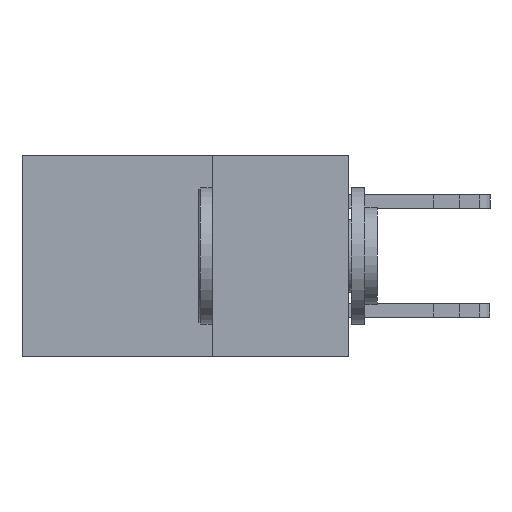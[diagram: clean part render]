
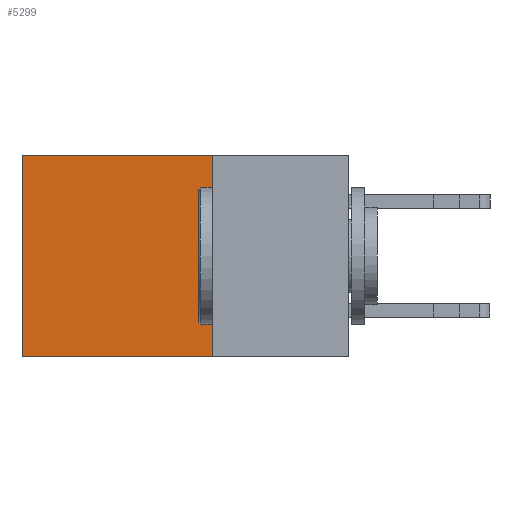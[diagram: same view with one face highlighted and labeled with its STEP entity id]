
A CAD part, left-side view. The second image highlights one B-rep face of the part: STEP entity #5299.
In plain terms, the highlighted planar face has unit normal (-1, 0, 0).
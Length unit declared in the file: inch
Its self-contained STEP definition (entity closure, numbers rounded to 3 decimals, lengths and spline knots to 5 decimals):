
#63 = CARTESIAN_POINT ( 'NONE',  ( 0.298, 0.6, -0.37 ) ) ;
#102 = CARTESIAN_POINT ( 'NONE',  ( 0.298, 0.25, 0. ) ) ;
#110 = ORIENTED_EDGE ( 'NONE', *, *, #8797, .F. ) ;
#428 = DIRECTION ( 'NONE',  ( 1., 0., 0. ) ) ;
#629 = CARTESIAN_POINT ( 'NONE',  ( 0.298, 0.25, 0. ) ) ;
#1063 = DIRECTION ( 'NONE',  ( 0., 0., -1. ) ) ;
#1557 = VERTEX_POINT ( 'NONE', #14944 ) ;
#1752 = VERTEX_POINT ( 'NONE', #15256 ) ;
#2557 = CARTESIAN_POINT ( 'NONE',  ( 0.298, 0.25, -0.37 ) ) ;
#2605 = EDGE_LOOP ( 'NONE', ( #8433, #110, #6598, #8859 ) ) ;
#3807 = EDGE_CURVE ( 'NONE', #1752, #10087, #8026, .T. ) ;
#3859 = VECTOR ( 'NONE', #1063, 39.37008 ) ;
#4350 = VECTOR ( 'NONE', #9693, 39.37008 ) ;
#4634 = VERTEX_POINT ( 'NONE', #63 ) ;
#4769 = EDGE_CURVE ( 'NONE', #1752, #1557, #9518, .T. ) ;
#5299 = ADVANCED_FACE ( 'NONE', ( #9339 ), #12120, .F. ) ;
#5301 = DIRECTION ( 'NONE',  ( 0., 1., 0. ) ) ;
#6598 = ORIENTED_EDGE ( 'NONE', *, *, #3807, .F. ) ;
#6764 = AXIS2_PLACEMENT_3D ( 'NONE', #629, #428, #7279 ) ;
#7110 = LINE ( 'NONE', #13192, #3859 ) ;
#7279 = DIRECTION ( 'NONE',  ( 0., 0., -1. ) ) ;
#8026 = LINE ( 'NONE', #9883, #4350 ) ;
#8433 = ORIENTED_EDGE ( 'NONE', *, *, #15404, .T. ) ;
#8797 = EDGE_CURVE ( 'NONE', #10087, #4634, #14707, .T. ) ;
#8854 = VECTOR ( 'NONE', #5301, 39.37008 ) ;
#8859 = ORIENTED_EDGE ( 'NONE', *, *, #4769, .T. ) ;
#9339 = FACE_OUTER_BOUND ( 'NONE', #2605, .T. ) ;
#9518 = LINE ( 'NONE', #102, #12253 ) ;
#9693 = DIRECTION ( 'NONE',  ( 0., 0., -1. ) ) ;
#9883 = CARTESIAN_POINT ( 'NONE',  ( 0.298, 0.25, 0. ) ) ;
#9946 = DIRECTION ( 'NONE',  ( 0., 1., 0. ) ) ;
#10087 = VERTEX_POINT ( 'NONE', #2557 ) ;
#12120 = PLANE ( 'NONE',  #6764 ) ;
#12253 = VECTOR ( 'NONE', #9946, 39.37008 ) ;
#13192 = CARTESIAN_POINT ( 'NONE',  ( 0.298, 0.6, 0. ) ) ;
#13743 = CARTESIAN_POINT ( 'NONE',  ( 0.298, 0.25, -0.37 ) ) ;
#14707 = LINE ( 'NONE', #13743, #8854 ) ;
#14944 = CARTESIAN_POINT ( 'NONE',  ( 0.298, 0.6, 0. ) ) ;
#15256 = CARTESIAN_POINT ( 'NONE',  ( 0.298, 0.25, 0. ) ) ;
#15404 = EDGE_CURVE ( 'NONE', #1557, #4634, #7110, .T. ) ;
